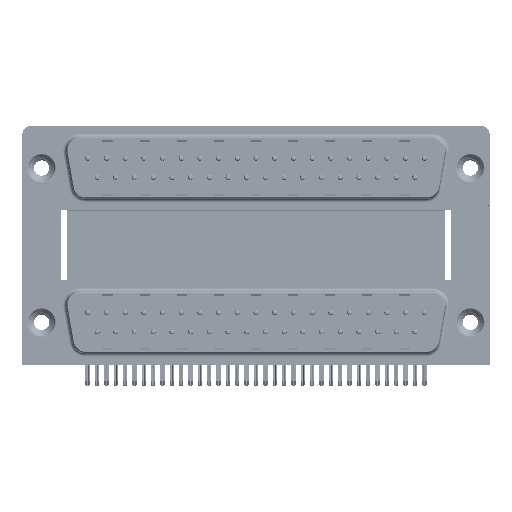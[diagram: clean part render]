
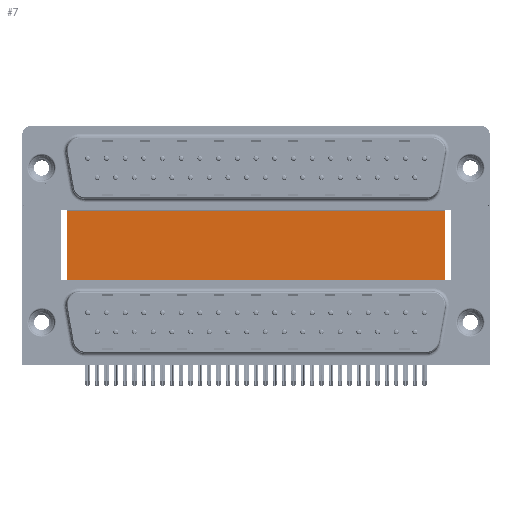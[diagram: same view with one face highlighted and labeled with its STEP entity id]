
A CAD part, top view. The second image highlights one B-rep face of the part: STEP entity #7.
In plain terms, the highlighted planar face has unit normal (0, 0, 1).
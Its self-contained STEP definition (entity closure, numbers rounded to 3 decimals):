
#7 = ADVANCED_FACE ( 'NONE', ( #26350 ), #49754, .F. ) ;
#1341 = EDGE_LOOP ( 'NONE', ( #13293, #48079, #39325, #40017 ) ) ;
#1682 = LINE ( 'NONE', #17366, #11558 ) ;
#2995 = DIRECTION ( 'NONE',  ( -1., 0., 0. ) ) ;
#3057 = EDGE_CURVE ( 'NONE', #23378, #24584, #32934, .T. ) ;
#3917 = AXIS2_PLACEMENT_3D ( 'NONE', #26107, #19433, #2995 ) ;
#5355 = VERTEX_POINT ( 'NONE', #14114 ) ;
#5488 = EDGE_CURVE ( 'NONE', #23378, #27930, #1682, .T. ) ;
#9206 = DIRECTION ( 'NONE',  ( 1., 0., 0. ) ) ;
#11558 = VECTOR ( 'NONE', #39940, 1000. ) ;
#13293 = ORIENTED_EDGE ( 'NONE', *, *, #47263, .T. ) ;
#13865 = CARTESIAN_POINT ( 'NONE',  ( 59.71, 16.585, -12. ) ) ;
#14114 = CARTESIAN_POINT ( 'NONE',  ( 59.71, -3.735, -12. ) ) ;
#17218 = EDGE_CURVE ( 'NONE', #27930, #5355, #19468, .T. ) ;
#17366 = CARTESIAN_POINT ( 'NONE',  ( 3.79, 16.585, -12. ) ) ;
#19433 = DIRECTION ( 'NONE',  ( 0., 0., -1. ) ) ;
#19468 = LINE ( 'NONE', #39451, #49194 ) ;
#21398 = CARTESIAN_POINT ( 'NONE',  ( 3.79, 16.585, -12. ) ) ;
#23378 = VERTEX_POINT ( 'NONE', #43214 ) ;
#24108 = CARTESIAN_POINT ( 'NONE',  ( 3.79, -3.735, -12. ) ) ;
#24584 = VERTEX_POINT ( 'NONE', #24108 ) ;
#26107 = CARTESIAN_POINT ( 'NONE',  ( 3.79, 16.585, -12. ) ) ;
#26350 = FACE_OUTER_BOUND ( 'NONE', #1341, .T. ) ;
#27930 = VERTEX_POINT ( 'NONE', #13865 ) ;
#32934 = LINE ( 'NONE', #21398, #47450 ) ;
#39317 = LINE ( 'NONE', #48250, #40326 ) ;
#39325 = ORIENTED_EDGE ( 'NONE', *, *, #5488, .F. ) ;
#39451 = CARTESIAN_POINT ( 'NONE',  ( 59.71, 16.585, -12. ) ) ;
#39940 = DIRECTION ( 'NONE',  ( 1., 0., 0. ) ) ;
#40017 = ORIENTED_EDGE ( 'NONE', *, *, #3057, .T. ) ;
#40326 = VECTOR ( 'NONE', #9206, 1000. ) ;
#43068 = DIRECTION ( 'NONE',  ( 0., -1., 0. ) ) ;
#43214 = CARTESIAN_POINT ( 'NONE',  ( 3.79, 16.585, -12. ) ) ;
#47263 = EDGE_CURVE ( 'NONE', #24584, #5355, #39317, .T. ) ;
#47450 = VECTOR ( 'NONE', #48383, 1000. ) ;
#48079 = ORIENTED_EDGE ( 'NONE', *, *, #17218, .F. ) ;
#48250 = CARTESIAN_POINT ( 'NONE',  ( 3.79, -3.735, -12. ) ) ;
#48383 = DIRECTION ( 'NONE',  ( 0., -1., 0. ) ) ;
#49194 = VECTOR ( 'NONE', #43068, 1000. ) ;
#49754 = PLANE ( 'NONE',  #3917 ) ;
